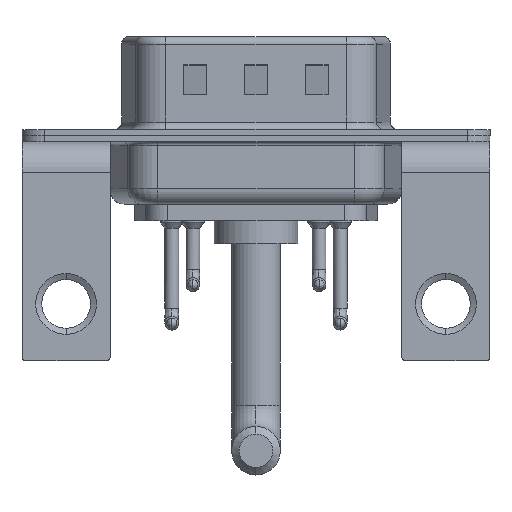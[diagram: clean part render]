
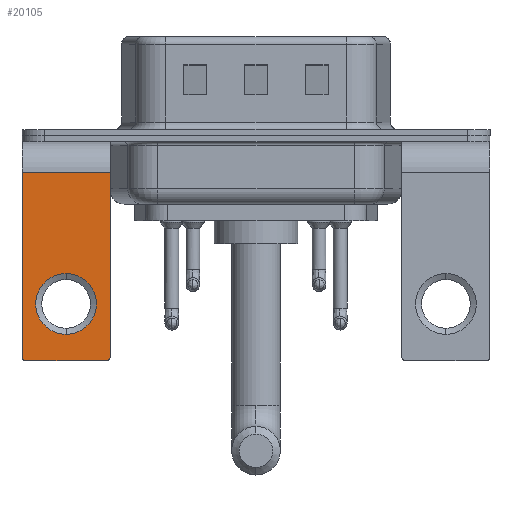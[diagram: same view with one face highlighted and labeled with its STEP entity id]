
A CAD part, front view. The second image highlights one B-rep face of the part: STEP entity #20105.
In plain terms, the highlighted planar face has unit normal (0, -1, 0).
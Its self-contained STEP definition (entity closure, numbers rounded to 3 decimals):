
#66 = DIRECTION ( 'NONE',  ( 0., -1., 0. ) ) ;
#263 = CIRCLE ( 'NONE', #10032, 0.25 ) ;
#395 = VERTEX_POINT ( 'NONE', #8607 ) ;
#634 = EDGE_CURVE ( 'NONE', #10148, #14024, #7878, .T. ) ;
#802 = DIRECTION ( 'NONE',  ( 0., 0., 1. ) ) ;
#1021 = CARTESIAN_POINT ( 'NONE',  ( -2.9, -6.25, -2.4 ) ) ;
#1415 = DIRECTION ( 'NONE',  ( 0., -1., 0. ) ) ;
#1416 = EDGE_CURVE ( 'NONE', #20059, #10125, #5990, .T. ) ;
#1724 = CARTESIAN_POINT ( 'NONE',  ( -2.9, -6.25, -2.4 ) ) ;
#2047 = CARTESIAN_POINT ( 'NONE',  ( 2.65, -6.25, -14.8 ) ) ;
#2231 = VERTEX_POINT ( 'NONE', #1021 ) ;
#2440 = ORIENTED_EDGE ( 'NONE', *, *, #7055, .T. ) ;
#2986 = VECTOR ( 'NONE', #6018, 1000. ) ;
#3008 = CARTESIAN_POINT ( 'NONE',  ( -2.9, -6.25, -14.55 ) ) ;
#3090 = CARTESIAN_POINT ( 'NONE',  ( 2.9, -6.25, -14.8 ) ) ;
#3545 = CIRCLE ( 'NONE', #17512, 2. ) ;
#4446 = CARTESIAN_POINT ( 'NONE',  ( -2.65, -6.25, -14.55 ) ) ;
#4597 = LINE ( 'NONE', #1724, #2986 ) ;
#4781 = DIRECTION ( 'NONE',  ( 0., 0., 1. ) ) ;
#4796 = VERTEX_POINT ( 'NONE', #3008 ) ;
#5136 = CARTESIAN_POINT ( 'NONE',  ( 2.9, -6.25, -2.4 ) ) ;
#5990 = LINE ( 'NONE', #12189, #19926 ) ;
#6018 = DIRECTION ( 'NONE',  ( 0., 0., -1. ) ) ;
#6086 = CIRCLE ( 'NONE', #11599, 2. ) ;
#6100 = ORIENTED_EDGE ( 'NONE', *, *, #9321, .T. ) ;
#7055 = EDGE_CURVE ( 'NONE', #20059, #2231, #17537, .T. ) ;
#7597 = DIRECTION ( 'NONE',  ( 0., 0., 1. ) ) ;
#7878 = LINE ( 'NONE', #3090, #18857 ) ;
#8158 = AXIS2_PLACEMENT_3D ( 'NONE', #19824, #1415, #4781 ) ;
#8204 = EDGE_CURVE ( 'NONE', #4796, #14024, #263, .T. ) ;
#8553 = CARTESIAN_POINT ( 'NONE',  ( 0., -6.25, -11.07 ) ) ;
#8607 = CARTESIAN_POINT ( 'NONE',  ( 0., -6.25, -9.07 ) ) ;
#9321 = EDGE_CURVE ( 'NONE', #395, #13727, #3545, .T. ) ;
#9420 = DIRECTION ( 'NONE',  ( 0., 1., 0. ) ) ;
#10032 = AXIS2_PLACEMENT_3D ( 'NONE', #4446, #66, #17046 ) ;
#10125 = VERTEX_POINT ( 'NONE', #13127 ) ;
#10148 = VERTEX_POINT ( 'NONE', #2047 ) ;
#10317 = ORIENTED_EDGE ( 'NONE', *, *, #1416, .F. ) ;
#10755 = EDGE_CURVE ( 'NONE', #10148, #10125, #19489, .T. ) ;
#11239 = FACE_OUTER_BOUND ( 'NONE', #15416, .T. ) ;
#11599 = AXIS2_PLACEMENT_3D ( 'NONE', #8553, #19599, #802 ) ;
#12118 = EDGE_CURVE ( 'NONE', #2231, #4796, #4597, .T. ) ;
#12189 = CARTESIAN_POINT ( 'NONE',  ( 2.9, -6.25, -2.4 ) ) ;
#12351 = DIRECTION ( 'NONE',  ( -1., 0., 0. ) ) ;
#12380 = ORIENTED_EDGE ( 'NONE', *, *, #12118, .T. ) ;
#12525 = EDGE_CURVE ( 'NONE', #13727, #395, #6086, .T. ) ;
#12550 = ORIENTED_EDGE ( 'NONE', *, *, #10755, .T. ) ;
#13114 = EDGE_LOOP ( 'NONE', ( #20058, #6100 ) ) ;
#13127 = CARTESIAN_POINT ( 'NONE',  ( 2.9, -6.25, -14.55 ) ) ;
#13727 = VERTEX_POINT ( 'NONE', #16050 ) ;
#14024 = VERTEX_POINT ( 'NONE', #16547 ) ;
#14075 = DIRECTION ( 'NONE',  ( 0., 0., 1. ) ) ;
#14160 = CARTESIAN_POINT ( 'NONE',  ( 2.9, -6.25, -2.4 ) ) ;
#15416 = EDGE_LOOP ( 'NONE', ( #12380, #16918, #18972, #12550, #10317, #2440 ) ) ;
#15886 = PLANE ( 'NONE',  #16614 ) ;
#16050 = CARTESIAN_POINT ( 'NONE',  ( 0., -6.25, -13.07 ) ) ;
#16201 = CARTESIAN_POINT ( 'NONE',  ( 2.9, -6.25, -2.4 ) ) ;
#16547 = CARTESIAN_POINT ( 'NONE',  ( -2.65, -6.25, -14.8 ) ) ;
#16614 = AXIS2_PLACEMENT_3D ( 'NONE', #14160, #9420, #14075 ) ;
#16650 = DIRECTION ( 'NONE',  ( 0., 0., -1. ) ) ;
#16816 = CARTESIAN_POINT ( 'NONE',  ( 0., -6.25, -11.07 ) ) ;
#16918 = ORIENTED_EDGE ( 'NONE', *, *, #8204, .T. ) ;
#17046 = DIRECTION ( 'NONE',  ( 0., 0., 1. ) ) ;
#17221 = FACE_BOUND ( 'NONE', #13114, .T. ) ;
#17512 = AXIS2_PLACEMENT_3D ( 'NONE', #16816, #18446, #7597 ) ;
#17537 = LINE ( 'NONE', #16201, #19417 ) ;
#18446 = DIRECTION ( 'NONE',  ( 0., 1., 0. ) ) ;
#18857 = VECTOR ( 'NONE', #12351, 1000. ) ;
#18860 = DIRECTION ( 'NONE',  ( -1., 0., 0. ) ) ;
#18972 = ORIENTED_EDGE ( 'NONE', *, *, #634, .F. ) ;
#19417 = VECTOR ( 'NONE', #18860, 1000. ) ;
#19489 = CIRCLE ( 'NONE', #8158, 0.25 ) ;
#19599 = DIRECTION ( 'NONE',  ( 0., 1., 0. ) ) ;
#19824 = CARTESIAN_POINT ( 'NONE',  ( 2.65, -6.25, -14.55 ) ) ;
#19926 = VECTOR ( 'NONE', #16650, 1000. ) ;
#20058 = ORIENTED_EDGE ( 'NONE', *, *, #12525, .T. ) ;
#20059 = VERTEX_POINT ( 'NONE', #5136 ) ;
#20105 = ADVANCED_FACE ( 'NONE', ( #17221, #11239 ), #15886, .F. ) ;
